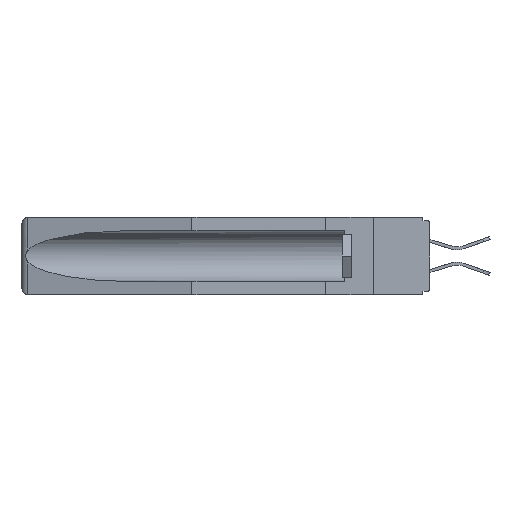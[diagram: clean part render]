
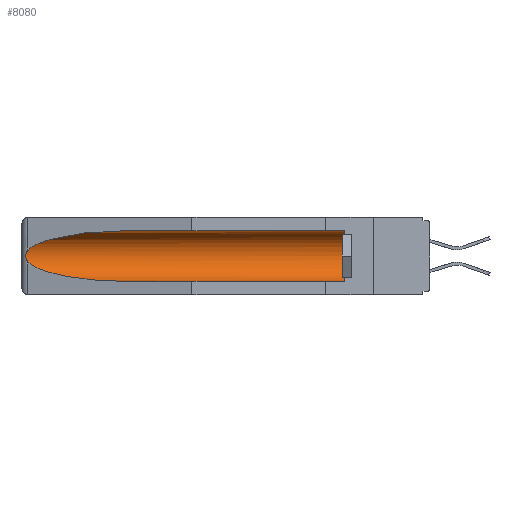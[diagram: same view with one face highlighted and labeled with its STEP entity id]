
A CAD part, left-side view. The second image highlights one B-rep face of the part: STEP entity #8080.
In plain terms, the highlighted cylindrical face has radius 2.857 mm (diameter 5.715 mm), a partial arc.
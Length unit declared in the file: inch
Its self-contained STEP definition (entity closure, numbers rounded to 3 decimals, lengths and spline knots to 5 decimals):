
#510 = VERTEX_POINT ( 'NONE', #17000 ) ;
#718 = CARTESIAN_POINT ( 'NONE',  ( 0.26537, 1.52718, -0.19328 ) ) ;
#759 = CARTESIAN_POINT ( 'NONE',  ( 0.155, 0.126, -0.059 ) ) ;
#792 = CARTESIAN_POINT ( 'NONE',  ( 0.155, 1.07973, -0.284 ) ) ;
#929 = ORIENTED_EDGE ( 'NONE', *, *, #13958, .T. ) ;
#1046 = CARTESIAN_POINT ( 'NONE',  ( 0.155, 0.126, -0.284 ) ) ;
#1863 = B_SPLINE_CURVE_WITH_KNOTS ( 'NONE', 3,
 ( #7624, #14140, #10625, #7419, #4100, #4177, #19139, #2323, #5682, #14000 ),
 .UNSPECIFIED., .F., .F.,
 ( 4, 2, 2, 2, 4 ),
 ( 0., 0.00029, 0.00058, 0.00087, 0.00117 ),
 .UNSPECIFIED. ) ;
#1954 = DIRECTION ( 'NONE',  ( 0., -1., 0. ) ) ;
#2170 = CARTESIAN_POINT ( 'NONE',  ( 0.26537, 1.52718, -0.14972 ) ) ;
#2186 = CARTESIAN_POINT ( 'NONE',  ( 0.26537, 1.52718, -0.19328 ) ) ;
#2323 = CARTESIAN_POINT ( 'NONE',  ( 0.26655, 1.53094, -0.18657 ) ) ;
#2450 = CARTESIAN_POINT ( 'NONE',  ( 0.25451, 1.48313, -0.09465 ) ) ;
#2460 = CARTESIAN_POINT ( 'NONE',  ( 0.25451, 1.48313, -0.24835 ) ) ;
#3298 = CARTESIAN_POINT ( 'NONE',  ( 0.155, -0.30754, -0.059 ) ) ;
#3375 = ORIENTED_EDGE ( 'NONE', *, *, #3865, .T. ) ;
#3865 = EDGE_CURVE ( 'NONE', #510, #5087, #13499, .T. ) ;
#4100 = CARTESIAN_POINT ( 'NONE',  ( 0.2675, 1.53308, -0.16763 ) ) ;
#4177 = CARTESIAN_POINT ( 'NONE',  ( 0.2675, 1.53308, -0.17534 ) ) ;
#4262 = CIRCLE ( 'NONE', #20551, 0.1125 ) ;
#4610 = CARTESIAN_POINT ( 'NONE',  ( 0.155, 1.07973, -0.284 ) ) ;
#4771 = EDGE_CURVE ( 'NONE', #13836, #13650, #4262, .T. ) ;
#5087 = VERTEX_POINT ( 'NONE', #14019 ) ;
#5140 = FACE_OUTER_BOUND ( 'NONE', #19229, .T. ) ;
#5682 = CARTESIAN_POINT ( 'NONE',  ( 0.26597, 1.5296, -0.19026 ) ) ;
#6121 = VECTOR ( 'NONE', #9537, 39.37008 ) ;
#6805 = CARTESIAN_POINT ( 'NONE',  ( 0.155, -0.30754, -0.284 ) ) ;
#7356 = VERTEX_POINT ( 'NONE', #2186 ) ;
#7419 = CARTESIAN_POINT ( 'NONE',  ( 0.2673, 1.5327, -0.16383 ) ) ;
#7624 = CARTESIAN_POINT ( 'NONE',  ( 0.26537, 1.52718, -0.14972 ) ) ;
#8080 = ADVANCED_FACE ( 'NONE', ( #5140 ), #20068, .F. ) ;
#8297 = ORIENTED_EDGE ( 'NONE', *, *, #15401, .T. ) ;
#8821 = EDGE_CURVE ( 'NONE', #5087, #7356, #1863, .T. ) ;
#8853 = DIRECTION ( 'NONE',  ( 0., 0., 1. ) ) ;
#9080 = CARTESIAN_POINT ( 'NONE',  ( 0.21114, 1.30732, -0.059 ) ) ;
#9254 = LINE ( 'NONE', #3298, #14475 ) ;
#9483 = EDGE_CURVE ( 'NONE', #13836, #20466, #14465, .T. ) ;
#9537 = DIRECTION ( 'NONE',  ( 0., 1., 0. ) ) ;
#10625 = CARTESIAN_POINT ( 'NONE',  ( 0.26654, 1.53092, -0.15636 ) ) ;
#12770 = ORIENTED_EDGE ( 'NONE', *, *, #8821, .T. ) ;
#13499 =( BOUNDED_CURVE ( )  B_SPLINE_CURVE ( 3, ( #14051, #9080, #2450, #2170 ),
 .UNSPECIFIED., .F., .F. ) 
 B_SPLINE_CURVE_WITH_KNOTS ( ( 4, 4 ),
 ( 4.71239, 6.08839 ),
 .UNSPECIFIED. ) 
 CURVE ( )  GEOMETRIC_REPRESENTATION_ITEM ( )  RATIONAL_B_SPLINE_CURVE ( ( 1., 0.848, 0.848, 1. ) ) 
 REPRESENTATION_ITEM ( '' )  );
#13551 = CARTESIAN_POINT ( 'NONE',  ( 0.155, -0.30754, -0.1715 ) ) ;
#13650 = VERTEX_POINT ( 'NONE', #759 ) ;
#13836 = VERTEX_POINT ( 'NONE', #1046 ) ;
#13958 = EDGE_CURVE ( 'NONE', #13650, #510, #9254, .T. ) ;
#14000 = CARTESIAN_POINT ( 'NONE',  ( 0.26537, 1.52718, -0.19328 ) ) ;
#14019 = CARTESIAN_POINT ( 'NONE',  ( 0.26537, 1.52718, -0.14972 ) ) ;
#14051 = CARTESIAN_POINT ( 'NONE',  ( 0.155, 1.07973, -0.059 ) ) ;
#14140 = CARTESIAN_POINT ( 'NONE',  ( 0.26597, 1.52961, -0.15275 ) ) ;
#14465 = LINE ( 'NONE', #6805, #6121 ) ;
#14475 = VECTOR ( 'NONE', #15044, 39.37008 ) ;
#15044 = DIRECTION ( 'NONE',  ( 0., 1., 0. ) ) ;
#15290 = CARTESIAN_POINT ( 'NONE',  ( 0.155, 0.126, -0.1715 ) ) ;
#15401 = EDGE_CURVE ( 'NONE', #7356, #20466, #21553, .T. ) ;
#16186 = ORIENTED_EDGE ( 'NONE', *, *, #9483, .F. ) ;
#17000 = CARTESIAN_POINT ( 'NONE',  ( 0.155, 1.07973, -0.059 ) ) ;
#18692 = DIRECTION ( 'NONE',  ( 0., 1., 0. ) ) ;
#18998 = CARTESIAN_POINT ( 'NONE',  ( 0.21114, 1.30732, -0.284 ) ) ;
#19139 = CARTESIAN_POINT ( 'NONE',  ( 0.2673, 1.53269, -0.17917 ) ) ;
#19229 = EDGE_LOOP ( 'NONE', ( #3375, #12770, #8297, #16186, #19762, #929 ) ) ;
#19762 = ORIENTED_EDGE ( 'NONE', *, *, #4771, .T. ) ;
#20012 = DIRECTION ( 'NONE',  ( 0., 0., 1. ) ) ;
#20068 = CYLINDRICAL_SURFACE ( 'NONE', #21289, 0.1125 ) ;
#20466 = VERTEX_POINT ( 'NONE', #4610 ) ;
#20551 = AXIS2_PLACEMENT_3D ( 'NONE', #15290, #1954, #8853 ) ;
#21289 = AXIS2_PLACEMENT_3D ( 'NONE', #13551, #18692, #20012 ) ;
#21553 =( BOUNDED_CURVE ( )  B_SPLINE_CURVE ( 3, ( #718, #2460, #18998, #792 ),
 .UNSPECIFIED., .F., .F. ) 
 B_SPLINE_CURVE_WITH_KNOTS ( ( 4, 4 ),
 ( 0.1948, 1.5708 ),
 .UNSPECIFIED. ) 
 CURVE ( )  GEOMETRIC_REPRESENTATION_ITEM ( )  RATIONAL_B_SPLINE_CURVE ( ( 1., 0.848, 0.848, 1. ) ) 
 REPRESENTATION_ITEM ( '' )  );
